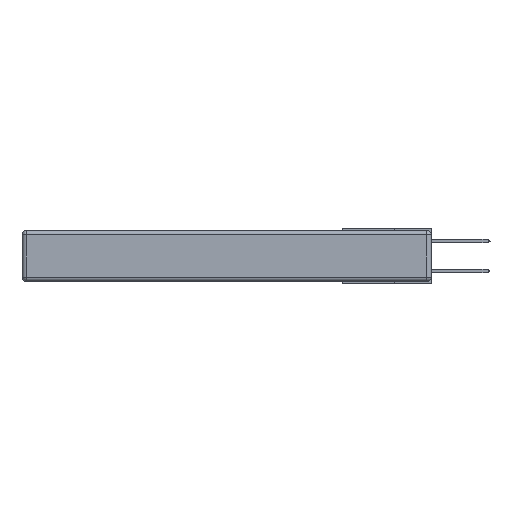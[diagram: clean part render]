
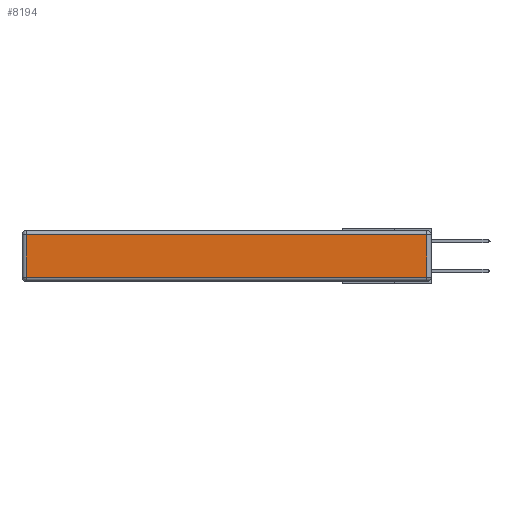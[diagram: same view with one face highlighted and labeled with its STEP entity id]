
A CAD part, left-side view. The second image highlights one B-rep face of the part: STEP entity #8194.
In plain terms, the highlighted planar face has unit normal (-1, 0, 0).
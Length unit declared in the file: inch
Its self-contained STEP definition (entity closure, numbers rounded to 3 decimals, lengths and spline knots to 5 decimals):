
#86 = LINE ( 'NONE', #1347, #10287 ) ;
#275 = CARTESIAN_POINT ( 'NONE',  ( 0., 0.03, -0.313 ) ) ;
#783 = ORIENTED_EDGE ( 'NONE', *, *, #7705, .T. ) ;
#1347 = CARTESIAN_POINT ( 'NONE',  ( 0., 0.03, -0.343 ) ) ;
#1751 = FACE_OUTER_BOUND ( 'NONE', #3900, .T. ) ;
#1914 = LINE ( 'NONE', #8642, #4029 ) ;
#2012 = CARTESIAN_POINT ( 'NONE',  ( 0., 2.72, -0.313 ) ) ;
#2216 = LINE ( 'NONE', #5669, #7527 ) ;
#3208 = ORIENTED_EDGE ( 'NONE', *, *, #7628, .T. ) ;
#3431 = DIRECTION ( 'NONE',  ( 0., -1., 0. ) ) ;
#3633 = CARTESIAN_POINT ( 'NONE',  ( 0., 2.75, -0.03 ) ) ;
#3792 = AXIS2_PLACEMENT_3D ( 'NONE', #9553, #11653, #7407 ) ;
#3900 = EDGE_LOOP ( 'NONE', ( #3208, #6457, #9075, #783 ) ) ;
#4029 = VECTOR ( 'NONE', #3431, 39.37008 ) ;
#4152 = EDGE_CURVE ( 'NONE', #4495, #11998, #9057, .T. ) ;
#4495 = VERTEX_POINT ( 'NONE', #10724 ) ;
#5669 = CARTESIAN_POINT ( 'NONE',  ( 0., 2.72, -0.343 ) ) ;
#6457 = ORIENTED_EDGE ( 'NONE', *, *, #8583, .T. ) ;
#6826 = DIRECTION ( 'NONE',  ( 0., 0., -1. ) ) ;
#7407 = DIRECTION ( 'NONE',  ( 0., 0., 1. ) ) ;
#7527 = VECTOR ( 'NONE', #6826, 39.37008 ) ;
#7628 = EDGE_CURVE ( 'NONE', #12539, #8912, #1914, .T. ) ;
#7705 = EDGE_CURVE ( 'NONE', #11998, #12539, #2216, .T. ) ;
#8194 = ADVANCED_FACE ( 'NONE', ( #1751 ), #9699, .T. ) ;
#8583 = EDGE_CURVE ( 'NONE', #8912, #4495, #86, .T. ) ;
#8642 = CARTESIAN_POINT ( 'NONE',  ( 0., 0., -0.313 ) ) ;
#8657 = DIRECTION ( 'NONE',  ( 0., 1., 0. ) ) ;
#8912 = VERTEX_POINT ( 'NONE', #275 ) ;
#9057 = LINE ( 'NONE', #3633, #12289 ) ;
#9075 = ORIENTED_EDGE ( 'NONE', *, *, #4152, .T. ) ;
#9553 = CARTESIAN_POINT ( 'NONE',  ( 0., 0., -0.343 ) ) ;
#9699 = PLANE ( 'NONE',  #3792 ) ;
#10287 = VECTOR ( 'NONE', #11840, 39.37008 ) ;
#10724 = CARTESIAN_POINT ( 'NONE',  ( 0., 0.03, -0.03 ) ) ;
#11634 = CARTESIAN_POINT ( 'NONE',  ( 0., 2.72, -0.03 ) ) ;
#11653 = DIRECTION ( 'NONE',  ( -1., 0., 0. ) ) ;
#11840 = DIRECTION ( 'NONE',  ( 0., 0., 1. ) ) ;
#11998 = VERTEX_POINT ( 'NONE', #11634 ) ;
#12289 = VECTOR ( 'NONE', #8657, 39.37008 ) ;
#12539 = VERTEX_POINT ( 'NONE', #2012 ) ;
